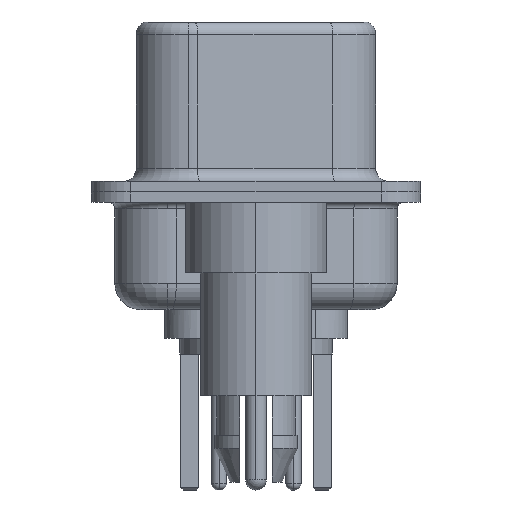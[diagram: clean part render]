
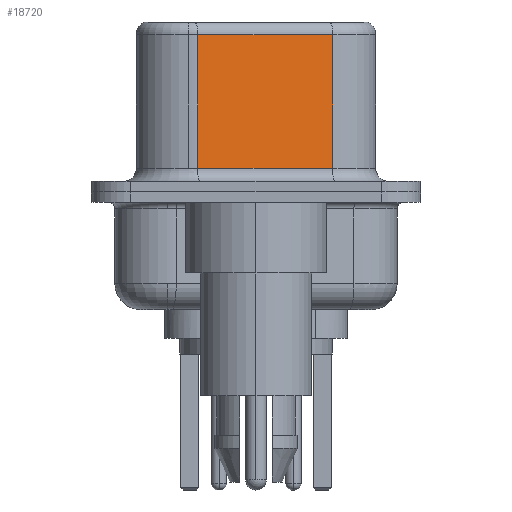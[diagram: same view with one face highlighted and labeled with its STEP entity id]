
A CAD part, left-side view. The second image highlights one B-rep face of the part: STEP entity #18720.
In plain terms, the highlighted planar face has unit normal (-0.985, -0.174, 0).
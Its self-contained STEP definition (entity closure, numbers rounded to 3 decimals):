
#1346 = CARTESIAN_POINT ( 'NONE',  ( 4.585, -2.927, 6.02 ) ) ;
#1966 = CARTESIAN_POINT ( 'NONE',  ( 4.585, -2.927, 0.9 ) ) ;
#2239 = DIRECTION ( 'NONE',  ( 0., 0., -1. ) ) ;
#2280 = ORIENTED_EDGE ( 'NONE', *, *, #9208, .T. ) ;
#2376 = DIRECTION ( 'NONE',  ( 0.174, -0.985, 0. ) ) ;
#3145 = EDGE_CURVE ( 'NONE', #6647, #3245, #5562, .T. ) ;
#3245 = VERTEX_POINT ( 'NONE', #4338 ) ;
#3549 = PLANE ( 'NONE',  #16511 ) ;
#3633 = CARTESIAN_POINT ( 'NONE',  ( 4.585, -2.927, 6.52 ) ) ;
#3647 = DIRECTION ( 'NONE',  ( 0., 0., -1. ) ) ;
#4142 = FACE_OUTER_BOUND ( 'NONE', #23152, .T. ) ;
#4338 = CARTESIAN_POINT ( 'NONE',  ( 3.675, 2.233, 0.9 ) ) ;
#4539 = LINE ( 'NONE', #6582, #17725 ) ;
#5393 = ORIENTED_EDGE ( 'NONE', *, *, #17114, .T. ) ;
#5562 = LINE ( 'NONE', #13383, #24456 ) ;
#5636 = VERTEX_POINT ( 'NONE', #1346 ) ;
#6582 = CARTESIAN_POINT ( 'NONE',  ( 4.585, -2.927, 6.02 ) ) ;
#6647 = VERTEX_POINT ( 'NONE', #12426 ) ;
#7405 = DIRECTION ( 'NONE',  ( 0.985, 0.174, 0. ) ) ;
#7422 = CARTESIAN_POINT ( 'NONE',  ( 4.585, -2.927, 6.52 ) ) ;
#8123 = LINE ( 'NONE', #23397, #8720 ) ;
#8720 = VECTOR ( 'NONE', #2376, 1000. ) ;
#9208 = EDGE_CURVE ( 'NONE', #5636, #6647, #4539, .T. ) ;
#9268 = ORIENTED_EDGE ( 'NONE', *, *, #23431, .F. ) ;
#11747 = ORIENTED_EDGE ( 'NONE', *, *, #3145, .T. ) ;
#12380 = DIRECTION ( 'NONE',  ( -0.174, 0.985, 0. ) ) ;
#12426 = CARTESIAN_POINT ( 'NONE',  ( 3.675, 2.233, 6.02 ) ) ;
#13016 = DIRECTION ( 'NONE',  ( -0.174, 0.985, 0. ) ) ;
#13262 = VERTEX_POINT ( 'NONE', #1966 ) ;
#13383 = CARTESIAN_POINT ( 'NONE',  ( 3.675, 2.233, 6.52 ) ) ;
#16242 = VECTOR ( 'NONE', #3647, 1000. ) ;
#16511 = AXIS2_PLACEMENT_3D ( 'NONE', #3633, #7405, #13016 ) ;
#17114 = EDGE_CURVE ( 'NONE', #3245, #13262, #8123, .T. ) ;
#17725 = VECTOR ( 'NONE', #12380, 1000. ) ;
#18720 = ADVANCED_FACE ( 'NONE', ( #4142 ), #3549, .F. ) ;
#18943 = LINE ( 'NONE', #7422, #16242 ) ;
#23152 = EDGE_LOOP ( 'NONE', ( #9268, #2280, #11747, #5393 ) ) ;
#23397 = CARTESIAN_POINT ( 'NONE',  ( 4.585, -2.927, 0.9 ) ) ;
#23431 = EDGE_CURVE ( 'NONE', #5636, #13262, #18943, .T. ) ;
#24456 = VECTOR ( 'NONE', #2239, 1000. ) ;
